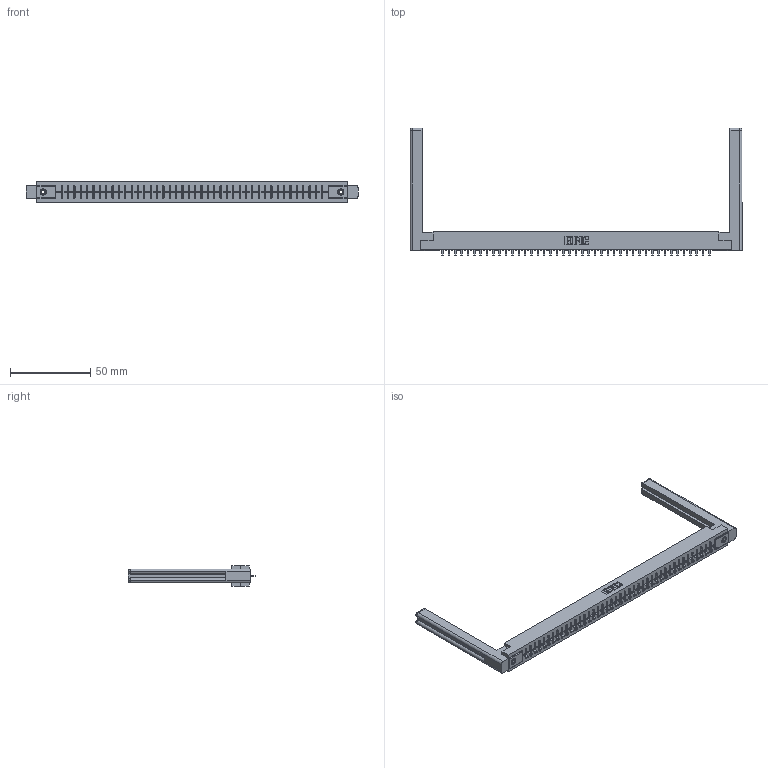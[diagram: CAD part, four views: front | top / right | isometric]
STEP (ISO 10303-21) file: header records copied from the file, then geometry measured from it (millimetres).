
FILE_DESCRIPTION (( 'STEP AP203' ), '1' );
FILE_NAME ('316-043-421-158.STEP', '2020-09-23T08:11:53', ( '' ), ( '' ), 'SwSTEP 2.0', 'SolidWorks 2020', '' );
FILE_SCHEMA (( 'CONFIG_CONTROL_DESIGN' ));
Length unit declared in the file: inch
Products named in the file (5): 316-043-421-158; 307-220-058; 306-290-001_121; 345-250-001_345-250-001-102; 306 Part_.156 Dia
Assembly tree (48 placements, depth 2):
  316-043-421-158
    306 Part_.156 Dia
    306-290-001_121  x43
    345-250-001_345-250-001-102  x2
    307-220-058  x2
Bounding box: 207.01 x 79.53 x 12.7 mm (x, y, z)
Volume: 29926.9 mm3; surface area: 28267.1 mm2
Topology: 48 solids, 48 shells, 3268 faces, 9141 edges, 5850 vertices
Faces by surface type: plane 2173, cylinder 899, sphere 172, cone 12, torus 12
Entity records: 42559 total; most frequent: CARTESIAN_POINT 7155, ORIENTED_EDGE 7036, DIRECTION 7010, EDGE_CURVE 3518, LINE 2748, VECTOR 2748, VERTEX_POINT 2222, AXIS2_PLACEMENT_3D 2131
